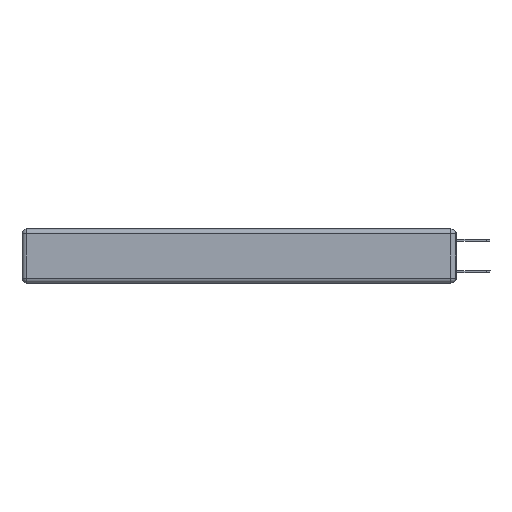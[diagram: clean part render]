
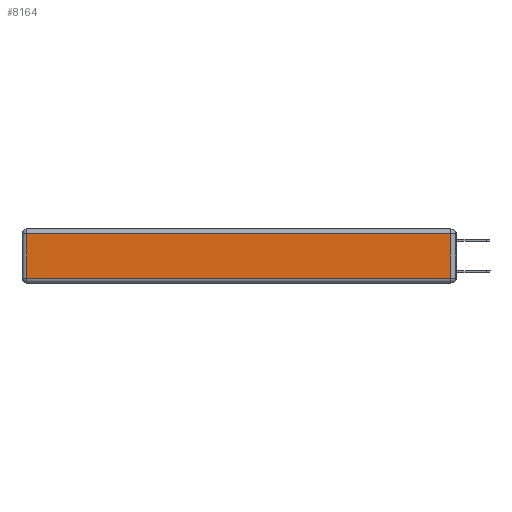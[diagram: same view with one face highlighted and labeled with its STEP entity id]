
A CAD part, left-side view. The second image highlights one B-rep face of the part: STEP entity #8164.
In plain terms, the highlighted planar face has unit normal (-1, 0, 0).
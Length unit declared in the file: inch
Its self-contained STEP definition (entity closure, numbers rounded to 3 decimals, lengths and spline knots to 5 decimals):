
#1661 = LINE ( 'NONE', #6741, #13478 ) ;
#2156 = CARTESIAN_POINT ( 'NONE',  ( 0., 0., -0.343 ) ) ;
#2481 = CARTESIAN_POINT ( 'NONE',  ( 0., 2.72, -0.343 ) ) ;
#3175 = ORIENTED_EDGE ( 'NONE', *, *, #10926, .T. ) ;
#3350 = DIRECTION ( 'NONE',  ( -1., 0., 0. ) ) ;
#3516 = VECTOR ( 'NONE', #10593, 39.37008 ) ;
#3869 = LINE ( 'NONE', #2481, #3516 ) ;
#4490 = LINE ( 'NONE', #7504, #12349 ) ;
#4735 = ORIENTED_EDGE ( 'NONE', *, *, #13609, .T. ) ;
#5231 = CARTESIAN_POINT ( 'NONE',  ( 0., 2.72, -0.03 ) ) ;
#5373 = EDGE_CURVE ( 'NONE', #9192, #12437, #4490, .T. ) ;
#5396 = ORIENTED_EDGE ( 'NONE', *, *, #11351, .T. ) ;
#5473 = LINE ( 'NONE', #5562, #6897 ) ;
#5562 = CARTESIAN_POINT ( 'NONE',  ( 0., 0.03, -0.343 ) ) ;
#6741 = CARTESIAN_POINT ( 'NONE',  ( 0., 2.75, -0.03 ) ) ;
#6897 = VECTOR ( 'NONE', #10140, 39.37008 ) ;
#7504 = CARTESIAN_POINT ( 'NONE',  ( 0., 0., -0.313 ) ) ;
#8164 = ADVANCED_FACE ( 'NONE', ( #14211 ), #13733, .T. ) ;
#8725 = CARTESIAN_POINT ( 'NONE',  ( 0., 0.03, -0.03 ) ) ;
#9191 = DIRECTION ( 'NONE',  ( 0., 0., 1. ) ) ;
#9192 = VERTEX_POINT ( 'NONE', #11907 ) ;
#9194 = DIRECTION ( 'NONE',  ( 0., 1., 0. ) ) ;
#9311 = ORIENTED_EDGE ( 'NONE', *, *, #5373, .T. ) ;
#10140 = DIRECTION ( 'NONE',  ( 0., 0., 1. ) ) ;
#10593 = DIRECTION ( 'NONE',  ( 0., 0., -1. ) ) ;
#10926 = EDGE_CURVE ( 'NONE', #12442, #9192, #3869, .T. ) ;
#11252 = VERTEX_POINT ( 'NONE', #8725 ) ;
#11351 = EDGE_CURVE ( 'NONE', #12437, #11252, #5473, .T. ) ;
#11462 = AXIS2_PLACEMENT_3D ( 'NONE', #2156, #3350, #9191 ) ;
#11907 = CARTESIAN_POINT ( 'NONE',  ( 0., 2.72, -0.313 ) ) ;
#12021 = CARTESIAN_POINT ( 'NONE',  ( 0., 0.03, -0.313 ) ) ;
#12349 = VECTOR ( 'NONE', #13193, 39.37008 ) ;
#12437 = VERTEX_POINT ( 'NONE', #12021 ) ;
#12442 = VERTEX_POINT ( 'NONE', #5231 ) ;
#13193 = DIRECTION ( 'NONE',  ( 0., -1., 0. ) ) ;
#13478 = VECTOR ( 'NONE', #9194, 39.37008 ) ;
#13609 = EDGE_CURVE ( 'NONE', #11252, #12442, #1661, .T. ) ;
#13733 = PLANE ( 'NONE',  #11462 ) ;
#14211 = FACE_OUTER_BOUND ( 'NONE', #14463, .T. ) ;
#14463 = EDGE_LOOP ( 'NONE', ( #9311, #5396, #4735, #3175 ) ) ;
